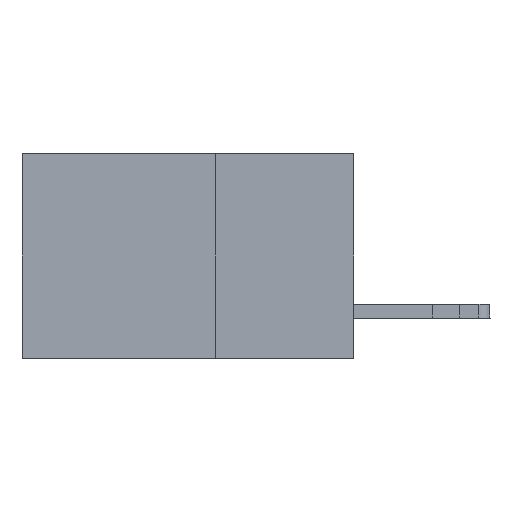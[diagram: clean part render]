
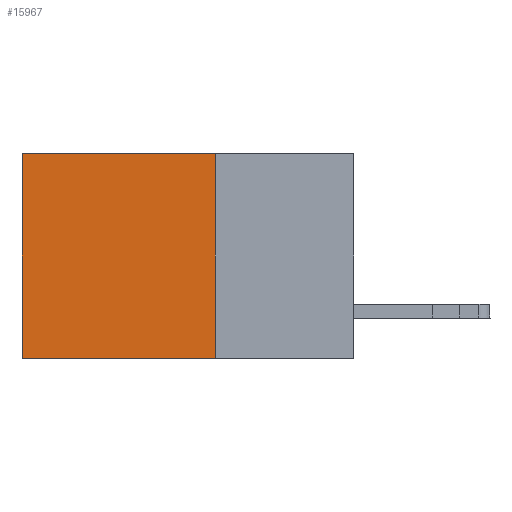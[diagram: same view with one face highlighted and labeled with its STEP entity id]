
A CAD part, left-side view. The second image highlights one B-rep face of the part: STEP entity #15967.
In plain terms, the highlighted planar face has unit normal (-1, 0, 0).
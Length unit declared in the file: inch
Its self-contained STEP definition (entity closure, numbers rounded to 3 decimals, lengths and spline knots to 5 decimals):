
#706 = ORIENTED_EDGE ( 'NONE', *, *, #21893, .F. ) ;
#1410 = VECTOR ( 'NONE', #10698, 39.37008 ) ;
#1724 = LINE ( 'NONE', #4809, #1410 ) ;
#2134 = EDGE_LOOP ( 'NONE', ( #17538, #706, #23671, #18660 ) ) ;
#2221 = DIRECTION ( 'NONE',  ( 0., 1., 0. ) ) ;
#2849 = DIRECTION ( 'NONE',  ( 0., 0., -1. ) ) ;
#2883 = VERTEX_POINT ( 'NONE', #4980 ) ;
#4109 = VECTOR ( 'NONE', #2849, 39.37008 ) ;
#4809 = CARTESIAN_POINT ( 'NONE',  ( 0.2875, 0.25, -0.37 ) ) ;
#4980 = CARTESIAN_POINT ( 'NONE',  ( 0.2875, 0.6, -0.37 ) ) ;
#5117 = CARTESIAN_POINT ( 'NONE',  ( 0.2875, 0.25, 0. ) ) ;
#6017 = DIRECTION ( 'NONE',  ( 0., 0., -1. ) ) ;
#6034 = EDGE_CURVE ( 'NONE', #19393, #2883, #12827, .T. ) ;
#6716 = VERTEX_POINT ( 'NONE', #5117 ) ;
#6925 = CARTESIAN_POINT ( 'NONE',  ( 0.2875, 0.25, 0. ) ) ;
#8700 = EDGE_CURVE ( 'NONE', #6716, #20777, #9928, .T. ) ;
#8899 = CARTESIAN_POINT ( 'NONE',  ( 0.2875, 0.6, 0. ) ) ;
#9677 = PLANE ( 'NONE',  #18913 ) ;
#9928 = LINE ( 'NONE', #6925, #4109 ) ;
#10698 = DIRECTION ( 'NONE',  ( 0., 1., 0. ) ) ;
#11259 = CARTESIAN_POINT ( 'NONE',  ( 0.2875, 0.25, 0. ) ) ;
#12827 = LINE ( 'NONE', #8899, #19945 ) ;
#13972 = VECTOR ( 'NONE', #2221, 39.37008 ) ;
#15967 = ADVANCED_FACE ( 'NONE', ( #22110 ), #9677, .F. ) ;
#17538 = ORIENTED_EDGE ( 'NONE', *, *, #6034, .T. ) ;
#17733 = DIRECTION ( 'NONE',  ( 1., 0., 0. ) ) ;
#18660 = ORIENTED_EDGE ( 'NONE', *, *, #20123, .T. ) ;
#18913 = AXIS2_PLACEMENT_3D ( 'NONE', #23468, #17733, #6017 ) ;
#19393 = VERTEX_POINT ( 'NONE', #20764 ) ;
#19945 = VECTOR ( 'NONE', #20697, 39.37008 ) ;
#20123 = EDGE_CURVE ( 'NONE', #6716, #19393, #20479, .T. ) ;
#20400 = CARTESIAN_POINT ( 'NONE',  ( 0.2875, 0.25, -0.37 ) ) ;
#20479 = LINE ( 'NONE', #11259, #13972 ) ;
#20697 = DIRECTION ( 'NONE',  ( 0., 0., -1. ) ) ;
#20764 = CARTESIAN_POINT ( 'NONE',  ( 0.2875, 0.6, 0. ) ) ;
#20777 = VERTEX_POINT ( 'NONE', #20400 ) ;
#21893 = EDGE_CURVE ( 'NONE', #20777, #2883, #1724, .T. ) ;
#22110 = FACE_OUTER_BOUND ( 'NONE', #2134, .T. ) ;
#23468 = CARTESIAN_POINT ( 'NONE',  ( 0.2875, 0.25, 0. ) ) ;
#23671 = ORIENTED_EDGE ( 'NONE', *, *, #8700, .F. ) ;
